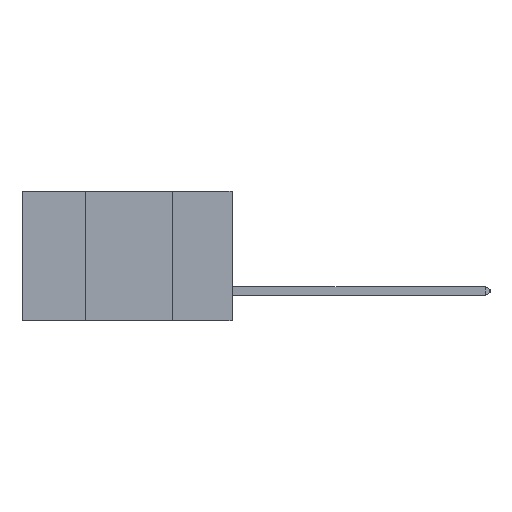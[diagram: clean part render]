
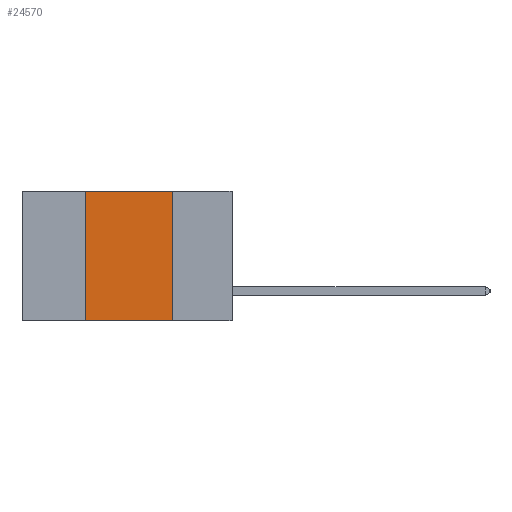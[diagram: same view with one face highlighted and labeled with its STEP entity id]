
A CAD part, left-side view. The second image highlights one B-rep face of the part: STEP entity #24570.
In plain terms, the highlighted planar face has unit normal (-1, 0, 0).
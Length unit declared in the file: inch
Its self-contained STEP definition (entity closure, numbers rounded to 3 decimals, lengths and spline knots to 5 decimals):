
#1464 = DIRECTION ( 'NONE',  ( 0., -1., 0. ) ) ;
#2197 = CARTESIAN_POINT ( 'NONE',  ( 0., 0.42, -0.37 ) ) ;
#2752 = ORIENTED_EDGE ( 'NONE', *, *, #11974, .F. ) ;
#3174 = ORIENTED_EDGE ( 'NONE', *, *, #23765, .F. ) ;
#3451 = LINE ( 'NONE', #17228, #31371 ) ;
#8654 = CARTESIAN_POINT ( 'NONE',  ( 0., 0.17, 0. ) ) ;
#9141 = VERTEX_POINT ( 'NONE', #33496 ) ;
#9449 = DIRECTION ( 'NONE',  ( 0., -1., 0. ) ) ;
#10835 = VECTOR ( 'NONE', #25977, 39.37008 ) ;
#10979 = PLANE ( 'NONE',  #32594 ) ;
#11077 = VERTEX_POINT ( 'NONE', #27939 ) ;
#11974 = EDGE_CURVE ( 'NONE', #11077, #9141, #25283, .T. ) ;
#15982 = VERTEX_POINT ( 'NONE', #2197 ) ;
#16279 = DIRECTION ( 'NONE',  ( 0., 0., -1. ) ) ;
#17228 = CARTESIAN_POINT ( 'NONE',  ( 0., 0.6, -0.37 ) ) ;
#17829 = LINE ( 'NONE', #33695, #10835 ) ;
#18242 = VERTEX_POINT ( 'NONE', #25012 ) ;
#18788 = CARTESIAN_POINT ( 'NONE',  ( 0., 0.6, 0. ) ) ;
#21147 = EDGE_CURVE ( 'NONE', #9141, #18242, #33555, .T. ) ;
#22542 = CARTESIAN_POINT ( 'NONE',  ( 0., 0.6, 0. ) ) ;
#23563 = EDGE_CURVE ( 'NONE', #15982, #18242, #3451, .T. ) ;
#23765 = EDGE_CURVE ( 'NONE', #15982, #11077, #17829, .T. ) ;
#24570 = ADVANCED_FACE ( 'NONE', ( #26398 ), #10979, .F. ) ;
#25012 = CARTESIAN_POINT ( 'NONE',  ( 0., 0.17, -0.37 ) ) ;
#25283 = LINE ( 'NONE', #22542, #33026 ) ;
#25977 = DIRECTION ( 'NONE',  ( 0., 0., 1. ) ) ;
#26398 = FACE_OUTER_BOUND ( 'NONE', #27233, .T. ) ;
#27021 = DIRECTION ( 'NONE',  ( 0., 0., -1. ) ) ;
#27233 = EDGE_LOOP ( 'NONE', ( #29009, #2752, #3174, #31144 ) ) ;
#27468 = VECTOR ( 'NONE', #27021, 39.37008 ) ;
#27939 = CARTESIAN_POINT ( 'NONE',  ( 0., 0.42, 0. ) ) ;
#29009 = ORIENTED_EDGE ( 'NONE', *, *, #21147, .F. ) ;
#31144 = ORIENTED_EDGE ( 'NONE', *, *, #23563, .T. ) ;
#31371 = VECTOR ( 'NONE', #1464, 39.37008 ) ;
#31960 = DIRECTION ( 'NONE',  ( 1., 0., 0. ) ) ;
#32594 = AXIS2_PLACEMENT_3D ( 'NONE', #18788, #31960, #16279 ) ;
#33026 = VECTOR ( 'NONE', #9449, 39.37008 ) ;
#33496 = CARTESIAN_POINT ( 'NONE',  ( 0., 0.17, 0. ) ) ;
#33555 = LINE ( 'NONE', #8654, #27468 ) ;
#33695 = CARTESIAN_POINT ( 'NONE',  ( 0., 0.42, 0. ) ) ;
